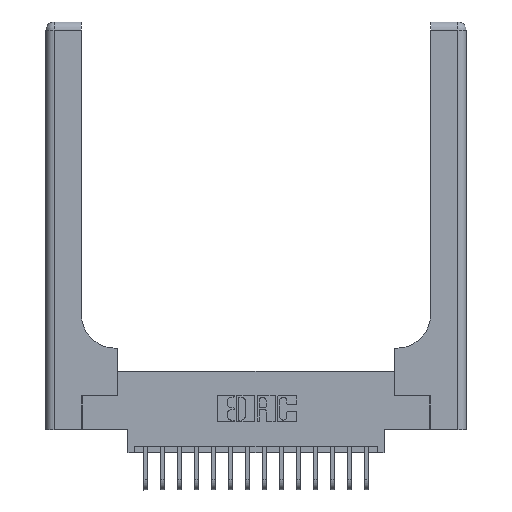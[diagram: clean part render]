
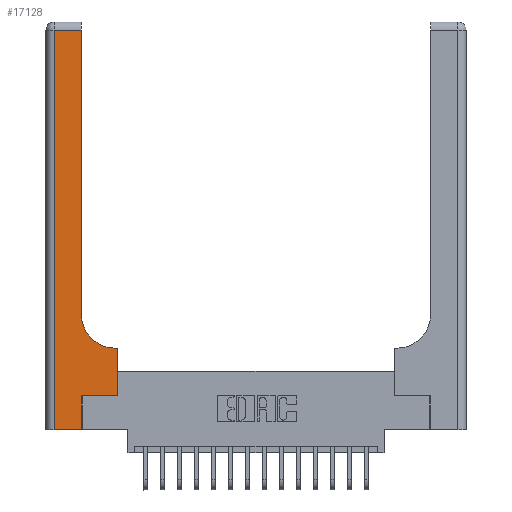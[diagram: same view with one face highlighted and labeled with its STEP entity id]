
A CAD part, top view. The second image highlights one B-rep face of the part: STEP entity #17128.
In plain terms, the highlighted planar face has unit normal (0, 0, 1).
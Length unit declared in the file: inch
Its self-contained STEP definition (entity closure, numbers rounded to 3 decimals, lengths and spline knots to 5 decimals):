
#130 = EDGE_CURVE ( 'NONE', #8281, #17584, #6601, .T. ) ;
#553 = LINE ( 'NONE', #18770, #13676 ) ;
#747 = VECTOR ( 'NONE', #7770, 39.37008 ) ;
#909 = VECTOR ( 'NONE', #16479, 39.37008 ) ;
#1286 = DIRECTION ( 'NONE',  ( -1., 0., 0. ) ) ;
#1392 = CARTESIAN_POINT ( 'NONE',  ( 0.26, 0.6, 0.37 ) ) ;
#1647 = VECTOR ( 'NONE', #18118, 39.37008 ) ;
#2071 = ORIENTED_EDGE ( 'NONE', *, *, #7026, .T. ) ;
#2315 = ORIENTED_EDGE ( 'NONE', *, *, #18491, .T. ) ;
#3014 = DIRECTION ( 'NONE',  ( -1., 0., 0. ) ) ;
#3132 = VECTOR ( 'NONE', #1286, 39.37008 ) ;
#3883 = ORIENTED_EDGE ( 'NONE', *, *, #19291, .T. ) ;
#4211 = AXIS2_PLACEMENT_3D ( 'NONE', #18168, #8907, #4279 ) ;
#4252 = VERTEX_POINT ( 'NONE', #5163 ) ;
#4279 = DIRECTION ( 'NONE',  ( 1., 0., 0. ) ) ;
#4653 = CARTESIAN_POINT ( 'NONE',  ( 0.265, 0.25, 0.37 ) ) ;
#4726 = PLANE ( 'NONE',  #16598 ) ;
#4911 = DIRECTION ( 'NONE',  ( 0., 1., 0. ) ) ;
#4984 = CIRCLE ( 'NONE', #4211, 0.25 ) ;
#5163 = CARTESIAN_POINT ( 'NONE',  ( 0.06, 0., 0.37 ) ) ;
#5319 = VERTEX_POINT ( 'NONE', #17045 ) ;
#5683 = VERTEX_POINT ( 'NONE', #15019 ) ;
#6224 = DIRECTION ( 'NONE',  ( -1., 0., 0. ) ) ;
#6299 = LINE ( 'NONE', #10517, #3132 ) ;
#6446 = ORIENTED_EDGE ( 'NONE', *, *, #16383, .T. ) ;
#6601 = LINE ( 'NONE', #7706, #747 ) ;
#6824 = LINE ( 'NONE', #14485, #10717 ) ;
#6952 = CARTESIAN_POINT ( 'NONE',  ( 0.528, 0.25, 0.37 ) ) ;
#7026 = EDGE_CURVE ( 'NONE', #5683, #11878, #553, .T. ) ;
#7706 = CARTESIAN_POINT ( 'NONE',  ( 0.528, 0.25, 0.37 ) ) ;
#7770 = DIRECTION ( 'NONE',  ( 0., 1., 0. ) ) ;
#8148 = EDGE_CURVE ( 'NONE', #16984, #10674, #6824, .T. ) ;
#8281 = VERTEX_POINT ( 'NONE', #6952 ) ;
#8907 = DIRECTION ( 'NONE',  ( 0., 0., -1. ) ) ;
#9058 = CARTESIAN_POINT ( 'NONE',  ( 0.528, 0.6, 0.37 ) ) ;
#9060 = CARTESIAN_POINT ( 'NONE',  ( 0., 0., 0.37 ) ) ;
#10240 = CARTESIAN_POINT ( 'NONE',  ( 0.265, 0.25, 0.37 ) ) ;
#10403 = ORIENTED_EDGE ( 'NONE', *, *, #17082, .T. ) ;
#10500 = VERTEX_POINT ( 'NONE', #11901 ) ;
#10517 = CARTESIAN_POINT ( 'NONE',  ( 0., 2.94, 0.37 ) ) ;
#10674 = VERTEX_POINT ( 'NONE', #17232 ) ;
#10717 = VECTOR ( 'NONE', #17459, 39.37008 ) ;
#10827 = EDGE_LOOP ( 'NONE', ( #10846, #6446, #15763, #3883, #2071, #2315, #10871, #10403, #15772 ) ) ;
#10846 = ORIENTED_EDGE ( 'NONE', *, *, #8148, .T. ) ;
#10871 = ORIENTED_EDGE ( 'NONE', *, *, #130, .T. ) ;
#11041 = DIRECTION ( 'NONE',  ( 0., 0., -1. ) ) ;
#11209 = EDGE_CURVE ( 'NONE', #10500, #4252, #11821, .T. ) ;
#11821 = LINE ( 'NONE', #13915, #17869 ) ;
#11878 = VERTEX_POINT ( 'NONE', #4653 ) ;
#11901 = CARTESIAN_POINT ( 'NONE',  ( 0.06, 2.94, 0.37 ) ) ;
#12528 = LINE ( 'NONE', #1392, #18960 ) ;
#12816 = EDGE_CURVE ( 'NONE', #5319, #16984, #4984, .T. ) ;
#13676 = VECTOR ( 'NONE', #4911, 39.37008 ) ;
#13915 = CARTESIAN_POINT ( 'NONE',  ( 0.06, 3., 0.37 ) ) ;
#14485 = CARTESIAN_POINT ( 'NONE',  ( 0.26, 3., 0.37 ) ) ;
#15019 = CARTESIAN_POINT ( 'NONE',  ( 0.265, 0., 0.37 ) ) ;
#15450 = FACE_OUTER_BOUND ( 'NONE', #10827, .T. ) ;
#15517 = CARTESIAN_POINT ( 'NONE',  ( 0., 3., 0.37 ) ) ;
#15533 = DIRECTION ( 'NONE',  ( 0., -1., 0. ) ) ;
#15713 = LINE ( 'NONE', #10240, #909 ) ;
#15763 = ORIENTED_EDGE ( 'NONE', *, *, #11209, .T. ) ;
#15772 = ORIENTED_EDGE ( 'NONE', *, *, #12816, .T. ) ;
#15971 = LINE ( 'NONE', #9060, #1647 ) ;
#16383 = EDGE_CURVE ( 'NONE', #10674, #10500, #6299, .T. ) ;
#16479 = DIRECTION ( 'NONE',  ( 1., 0., 0. ) ) ;
#16598 = AXIS2_PLACEMENT_3D ( 'NONE', #15517, #11041, #6224 ) ;
#16660 = CARTESIAN_POINT ( 'NONE',  ( 0.26, 0.85, 0.37 ) ) ;
#16984 = VERTEX_POINT ( 'NONE', #16660 ) ;
#17045 = CARTESIAN_POINT ( 'NONE',  ( 0.51, 0.6, 0.37 ) ) ;
#17082 = EDGE_CURVE ( 'NONE', #17584, #5319, #12528, .T. ) ;
#17128 = ADVANCED_FACE ( 'NONE', ( #15450 ), #4726, .F. ) ;
#17232 = CARTESIAN_POINT ( 'NONE',  ( 0.26, 2.94, 0.37 ) ) ;
#17459 = DIRECTION ( 'NONE',  ( 0., 1., 0. ) ) ;
#17584 = VERTEX_POINT ( 'NONE', #9058 ) ;
#17869 = VECTOR ( 'NONE', #15533, 39.37008 ) ;
#18118 = DIRECTION ( 'NONE',  ( 1., 0., 0. ) ) ;
#18168 = CARTESIAN_POINT ( 'NONE',  ( 0.51, 0.85, 0.37 ) ) ;
#18491 = EDGE_CURVE ( 'NONE', #11878, #8281, #15713, .T. ) ;
#18770 = CARTESIAN_POINT ( 'NONE',  ( 0.265, 0., 0.37 ) ) ;
#18960 = VECTOR ( 'NONE', #3014, 39.37008 ) ;
#19291 = EDGE_CURVE ( 'NONE', #4252, #5683, #15971, .T. ) ;
